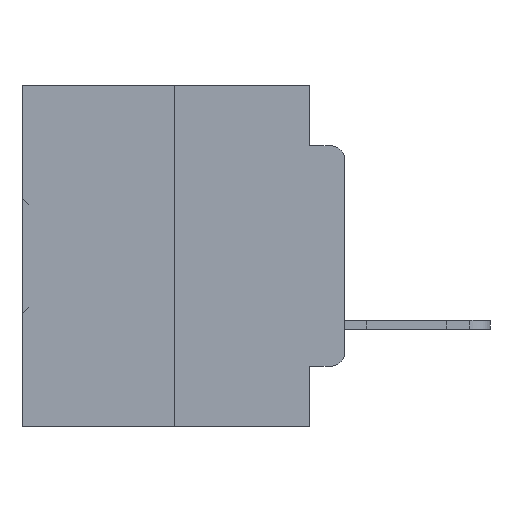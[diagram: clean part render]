
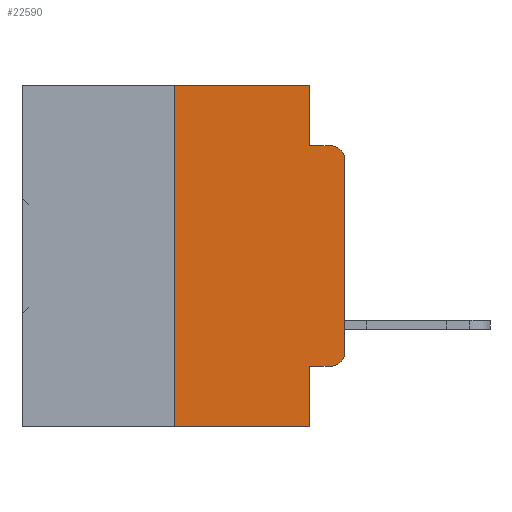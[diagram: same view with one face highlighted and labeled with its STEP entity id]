
A CAD part, left-side view. The second image highlights one B-rep face of the part: STEP entity #22590.
In plain terms, the highlighted planar face has unit normal (-1, 0, 0).
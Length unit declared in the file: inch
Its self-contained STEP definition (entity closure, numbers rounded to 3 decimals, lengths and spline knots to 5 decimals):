
#232 = LINE ( 'NONE', #9219, #14255 ) ;
#558 = CARTESIAN_POINT ( 'NONE',  ( 0., 0.473, 0. ) ) ;
#1122 = CARTESIAN_POINT ( 'NONE',  ( 0., 0.02, -0.4115 ) ) ;
#1505 = VERTEX_POINT ( 'NONE', #1122 ) ;
#2135 = CARTESIAN_POINT ( 'NONE',  ( 0., 0.473, -0.5 ) ) ;
#2448 = LINE ( 'NONE', #30983, #31634 ) ;
#2551 = EDGE_CURVE ( 'NONE', #36455, #24303, #24361, .T. ) ;
#3074 = DIRECTION ( 'NONE',  ( -1., 0., 0. ) ) ;
#3704 = ORIENTED_EDGE ( 'NONE', *, *, #11794, .T. ) ;
#3827 = EDGE_CURVE ( 'NONE', #8170, #28448, #19287, .T. ) ;
#4303 = AXIS2_PLACEMENT_3D ( 'NONE', #5913, #26339, #8898 ) ;
#4861 = LINE ( 'NONE', #2135, #20097 ) ;
#4897 = CARTESIAN_POINT ( 'NONE',  ( 0., 0.051, -0.4115 ) ) ;
#4974 = CARTESIAN_POINT ( 'NONE',  ( 0., 0.473, 0. ) ) ;
#5195 = DIRECTION ( 'NONE',  ( 0., -1., 0. ) ) ;
#5289 = CARTESIAN_POINT ( 'NONE',  ( 0., 0.25, -0.5 ) ) ;
#5733 = EDGE_CURVE ( 'NONE', #10304, #28448, #4861, .T. ) ;
#5913 = CARTESIAN_POINT ( 'NONE',  ( 0., 0.02, -0.1085 ) ) ;
#7978 = DIRECTION ( 'NONE',  ( 0., 0., -1. ) ) ;
#8170 = VERTEX_POINT ( 'NONE', #4897 ) ;
#8590 = DIRECTION ( 'NONE',  ( 0., 0., -1. ) ) ;
#8624 = VERTEX_POINT ( 'NONE', #23831 ) ;
#8762 = CARTESIAN_POINT ( 'NONE',  ( 0., 0.051, 0. ) ) ;
#8898 = DIRECTION ( 'NONE',  ( 0., 0., -1. ) ) ;
#9219 = CARTESIAN_POINT ( 'NONE',  ( 0., 0., 0. ) ) ;
#9243 = CARTESIAN_POINT ( 'NONE',  ( 0., 0.051, -0.4115 ) ) ;
#9851 = EDGE_CURVE ( 'NONE', #8170, #1505, #31401, .T. ) ;
#10304 = VERTEX_POINT ( 'NONE', #5289 ) ;
#10538 = VECTOR ( 'NONE', #24287, 39.37008 ) ;
#10614 = VECTOR ( 'NONE', #8590, 39.37008 ) ;
#11084 = ORIENTED_EDGE ( 'NONE', *, *, #35748, .F. ) ;
#11110 = ORIENTED_EDGE ( 'NONE', *, *, #3827, .F. ) ;
#11478 = ORIENTED_EDGE ( 'NONE', *, *, #2551, .F. ) ;
#11794 = EDGE_CURVE ( 'NONE', #1505, #30626, #35349, .T. ) ;
#12447 = ORIENTED_EDGE ( 'NONE', *, *, #5733, .T. ) ;
#14255 = VECTOR ( 'NONE', #32339, 39.37008 ) ;
#14479 = EDGE_CURVE ( 'NONE', #8624, #36455, #33608, .T. ) ;
#16225 = ORIENTED_EDGE ( 'NONE', *, *, #32594, .T. ) ;
#16646 = VECTOR ( 'NONE', #35936, 39.37008 ) ;
#16907 = EDGE_LOOP ( 'NONE', ( #22543, #16225, #11478, #36297, #35469, #11084, #12447, #11110, #19342, #3704 ) ) ;
#17872 = VECTOR ( 'NONE', #18345, 39.37008 ) ;
#18345 = DIRECTION ( 'NONE',  ( 0., -1., 0. ) ) ;
#18801 = LINE ( 'NONE', #558, #17872 ) ;
#18991 = CARTESIAN_POINT ( 'NONE',  ( 0., 0.02, -0.0885 ) ) ;
#19287 = LINE ( 'NONE', #8762, #10614 ) ;
#19342 = ORIENTED_EDGE ( 'NONE', *, *, #9851, .T. ) ;
#20097 = VECTOR ( 'NONE', #5195, 39.37008 ) ;
#20698 = CARTESIAN_POINT ( 'NONE',  ( 0., 0., -0.3915 ) ) ;
#20710 = CARTESIAN_POINT ( 'NONE',  ( 0., 0.02, -0.3915 ) ) ;
#21392 = CARTESIAN_POINT ( 'NONE',  ( 0., 0.051, 0. ) ) ;
#22543 = ORIENTED_EDGE ( 'NONE', *, *, #30661, .T. ) ;
#22545 = CARTESIAN_POINT ( 'NONE',  ( 0., 0., -0.1085 ) ) ;
#22590 = ADVANCED_FACE ( 'NONE', ( #30037 ), #36809, .F. ) ;
#23595 = DIRECTION ( 'NONE',  ( 0., 0., -1. ) ) ;
#23677 = AXIS2_PLACEMENT_3D ( 'NONE', #20710, #3074, #23595 ) ;
#23831 = CARTESIAN_POINT ( 'NONE',  ( 0., 0.051, 0. ) ) ;
#24287 = DIRECTION ( 'NONE',  ( 0., 0., -1. ) ) ;
#24303 = VERTEX_POINT ( 'NONE', #18991 ) ;
#24361 = LINE ( 'NONE', #35984, #16646 ) ;
#25428 = DIRECTION ( 'NONE',  ( 1., 0., 0. ) ) ;
#25628 = VECTOR ( 'NONE', #29475, 39.37008 ) ;
#25676 = CIRCLE ( 'NONE', #4303, 0.02 ) ;
#26339 = DIRECTION ( 'NONE',  ( -1., 0., 0. ) ) ;
#28383 = VERTEX_POINT ( 'NONE', #29739 ) ;
#28448 = VERTEX_POINT ( 'NONE', #33016 ) ;
#29475 = DIRECTION ( 'NONE',  ( 0., -1., 0. ) ) ;
#29739 = CARTESIAN_POINT ( 'NONE',  ( 0., 0.25, 0. ) ) ;
#30037 = FACE_OUTER_BOUND ( 'NONE', #16907, .T. ) ;
#30419 = AXIS2_PLACEMENT_3D ( 'NONE', #4974, #25428, #7978 ) ;
#30626 = VERTEX_POINT ( 'NONE', #20698 ) ;
#30661 = EDGE_CURVE ( 'NONE', #30626, #32426, #232, .T. ) ;
#30983 = CARTESIAN_POINT ( 'NONE',  ( 0., 0.25, 0. ) ) ;
#31018 = EDGE_CURVE ( 'NONE', #28383, #8624, #18801, .T. ) ;
#31401 = LINE ( 'NONE', #9243, #25628 ) ;
#31634 = VECTOR ( 'NONE', #33906, 39.37008 ) ;
#32339 = DIRECTION ( 'NONE',  ( 0., 0., 1. ) ) ;
#32426 = VERTEX_POINT ( 'NONE', #22545 ) ;
#32594 = EDGE_CURVE ( 'NONE', #32426, #24303, #25676, .T. ) ;
#33016 = CARTESIAN_POINT ( 'NONE',  ( 0., 0.051, -0.5 ) ) ;
#33608 = LINE ( 'NONE', #21392, #10538 ) ;
#33906 = DIRECTION ( 'NONE',  ( 0., 0., 1. ) ) ;
#34113 = CARTESIAN_POINT ( 'NONE',  ( 0., 0.051, -0.0885 ) ) ;
#35349 = CIRCLE ( 'NONE', #23677, 0.02 ) ;
#35469 = ORIENTED_EDGE ( 'NONE', *, *, #31018, .F. ) ;
#35748 = EDGE_CURVE ( 'NONE', #10304, #28383, #2448, .T. ) ;
#35936 = DIRECTION ( 'NONE',  ( 0., -1., 0. ) ) ;
#35984 = CARTESIAN_POINT ( 'NONE',  ( 0., 0.051, -0.0885 ) ) ;
#36297 = ORIENTED_EDGE ( 'NONE', *, *, #14479, .F. ) ;
#36455 = VERTEX_POINT ( 'NONE', #34113 ) ;
#36809 = PLANE ( 'NONE',  #30419 ) ;
